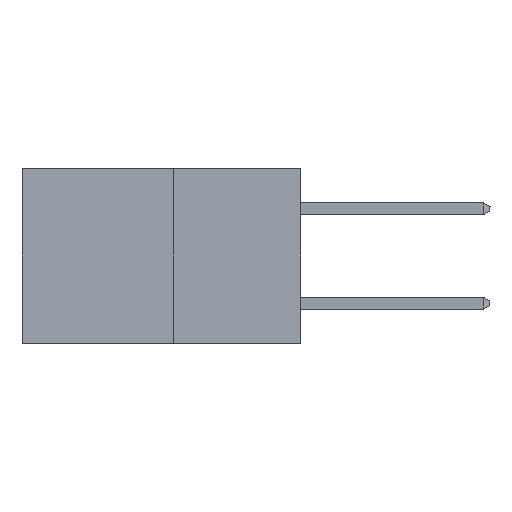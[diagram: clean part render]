
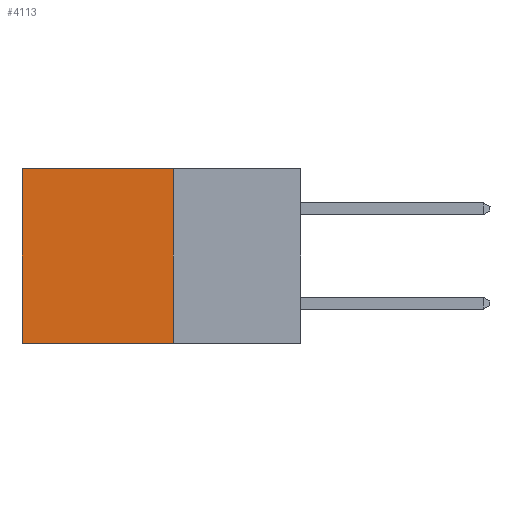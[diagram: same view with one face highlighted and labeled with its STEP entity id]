
A CAD part, left-side view. The second image highlights one B-rep face of the part: STEP entity #4113.
In plain terms, the highlighted planar face has unit normal (-1, 0, 0).
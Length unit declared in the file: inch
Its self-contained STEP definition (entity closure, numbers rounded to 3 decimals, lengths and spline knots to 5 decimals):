
#231 = VERTEX_POINT ( 'NONE', #7524 ) ;
#337 = ORIENTED_EDGE ( 'NONE', *, *, #5220, .T. ) ;
#451 = CARTESIAN_POINT ( 'NONE',  ( 0.277, 0.59, -0.37 ) ) ;
#1027 = EDGE_CURVE ( 'NONE', #3062, #3799, #6336, .T. ) ;
#1057 = DIRECTION ( 'NONE',  ( 0., 0., -1. ) ) ;
#1506 = ORIENTED_EDGE ( 'NONE', *, *, #2912, .T. ) ;
#1635 = CARTESIAN_POINT ( 'NONE',  ( 0.277, 0.27, -0.37 ) ) ;
#1748 = DIRECTION ( 'NONE',  ( 0., 0., -1. ) ) ;
#1776 = CARTESIAN_POINT ( 'NONE',  ( 0.277, 0.27, 0. ) ) ;
#1796 = LINE ( 'NONE', #6233, #7713 ) ;
#2105 = EDGE_LOOP ( 'NONE', ( #1506, #9596, #9812, #337 ) ) ;
#2187 = VECTOR ( 'NONE', #9617, 39.37008 ) ;
#2912 = EDGE_CURVE ( 'NONE', #231, #3799, #8273, .T. ) ;
#3062 = VERTEX_POINT ( 'NONE', #3933 ) ;
#3512 = EDGE_CURVE ( 'NONE', #3794, #3062, #9099, .T. ) ;
#3613 = FACE_OUTER_BOUND ( 'NONE', #2105, .T. ) ;
#3794 = VERTEX_POINT ( 'NONE', #1776 ) ;
#3799 = VERTEX_POINT ( 'NONE', #4167 ) ;
#3933 = CARTESIAN_POINT ( 'NONE',  ( 0.277, 0.27, -0.37 ) ) ;
#4024 = DIRECTION ( 'NONE',  ( 0., 0., -1. ) ) ;
#4113 = ADVANCED_FACE ( 'NONE', ( #3613 ), #6054, .F. ) ;
#4167 = CARTESIAN_POINT ( 'NONE',  ( 0.277, 0.59, -0.37 ) ) ;
#4942 = DIRECTION ( 'NONE',  ( 1., 0., 0. ) ) ;
#5220 = EDGE_CURVE ( 'NONE', #3794, #231, #1796, .T. ) ;
#5885 = CARTESIAN_POINT ( 'NONE',  ( 0.277, 0.27, -0.37 ) ) ;
#6054 = PLANE ( 'NONE',  #6061 ) ;
#6061 = AXIS2_PLACEMENT_3D ( 'NONE', #1635, #4942, #4024 ) ;
#6221 = DIRECTION ( 'NONE',  ( 0., 1., 0. ) ) ;
#6233 = CARTESIAN_POINT ( 'NONE',  ( 0.277, 0.27, 0. ) ) ;
#6336 = LINE ( 'NONE', #5885, #2187 ) ;
#6393 = VECTOR ( 'NONE', #1057, 39.37008 ) ;
#6567 = CARTESIAN_POINT ( 'NONE',  ( 0.277, 0.27, -0.37 ) ) ;
#6963 = VECTOR ( 'NONE', #1748, 39.37008 ) ;
#7524 = CARTESIAN_POINT ( 'NONE',  ( 0.277, 0.59, 0. ) ) ;
#7713 = VECTOR ( 'NONE', #6221, 39.37008 ) ;
#8273 = LINE ( 'NONE', #451, #6393 ) ;
#9099 = LINE ( 'NONE', #6567, #6963 ) ;
#9596 = ORIENTED_EDGE ( 'NONE', *, *, #1027, .F. ) ;
#9617 = DIRECTION ( 'NONE',  ( 0., 1., 0. ) ) ;
#9812 = ORIENTED_EDGE ( 'NONE', *, *, #3512, .F. ) ;
